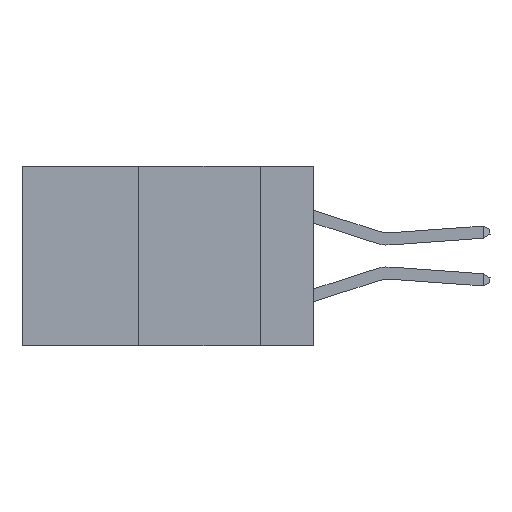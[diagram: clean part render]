
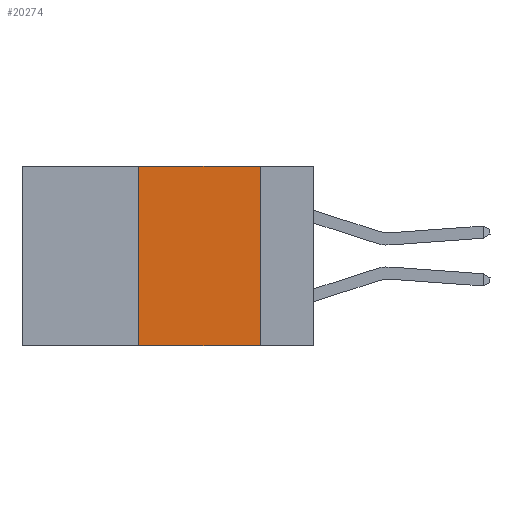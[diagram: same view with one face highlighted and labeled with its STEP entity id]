
A CAD part, left-side view. The second image highlights one B-rep face of the part: STEP entity #20274.
In plain terms, the highlighted planar face has unit normal (-1, 0, 0).
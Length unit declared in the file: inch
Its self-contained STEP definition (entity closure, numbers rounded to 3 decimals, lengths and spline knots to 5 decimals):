
#1145 = FACE_OUTER_BOUND ( 'NONE', #20582, .T. ) ;
#2050 = VERTEX_POINT ( 'NONE', #13366 ) ;
#3745 = ORIENTED_EDGE ( 'NONE', *, *, #16689, .F. ) ;
#4693 = LINE ( 'NONE', #27368, #33928 ) ;
#4699 = EDGE_CURVE ( 'NONE', #14085, #8470, #4693, .T. ) ;
#4722 = VECTOR ( 'NONE', #23053, 39.37008 ) ;
#7476 = CARTESIAN_POINT ( 'NONE',  ( 0., 0.11, 0. ) ) ;
#8258 = PLANE ( 'NONE',  #18762 ) ;
#8470 = VERTEX_POINT ( 'NONE', #16312 ) ;
#10323 = VECTOR ( 'NONE', #19302, 39.37008 ) ;
#13366 = CARTESIAN_POINT ( 'NONE',  ( 0., 0.11, 0. ) ) ;
#14085 = VERTEX_POINT ( 'NONE', #34231 ) ;
#14218 = CARTESIAN_POINT ( 'NONE',  ( 0., 0.6, 0. ) ) ;
#15478 = LINE ( 'NONE', #20334, #10323 ) ;
#15614 = LINE ( 'NONE', #22659, #30700 ) ;
#16303 = EDGE_CURVE ( 'NONE', #36599, #2050, #15614, .T. ) ;
#16312 = CARTESIAN_POINT ( 'NONE',  ( 0., 0.11, -0.37 ) ) ;
#16689 = EDGE_CURVE ( 'NONE', #2050, #8470, #35361, .T. ) ;
#18762 = AXIS2_PLACEMENT_3D ( 'NONE', #14218, #32512, #35388 ) ;
#19302 = DIRECTION ( 'NONE',  ( 0., 0., 1. ) ) ;
#20274 = ADVANCED_FACE ( 'NONE', ( #1145 ), #8258, .F. ) ;
#20334 = CARTESIAN_POINT ( 'NONE',  ( 0., 0.36, 0. ) ) ;
#20582 = EDGE_LOOP ( 'NONE', ( #3745, #25035, #38592, #24503 ) ) ;
#20878 = DIRECTION ( 'NONE',  ( 0., -1., 0. ) ) ;
#22211 = EDGE_CURVE ( 'NONE', #14085, #36599, #15478, .T. ) ;
#22659 = CARTESIAN_POINT ( 'NONE',  ( 0., 0.6, 0. ) ) ;
#22759 = CARTESIAN_POINT ( 'NONE',  ( 0., 0.36, 0. ) ) ;
#23053 = DIRECTION ( 'NONE',  ( 0., 0., -1. ) ) ;
#24503 = ORIENTED_EDGE ( 'NONE', *, *, #4699, .T. ) ;
#25035 = ORIENTED_EDGE ( 'NONE', *, *, #16303, .F. ) ;
#27368 = CARTESIAN_POINT ( 'NONE',  ( 0., 0.6, -0.37 ) ) ;
#28794 = DIRECTION ( 'NONE',  ( 0., -1., 0. ) ) ;
#30700 = VECTOR ( 'NONE', #28794, 39.37008 ) ;
#32512 = DIRECTION ( 'NONE',  ( 1., 0., 0. ) ) ;
#33928 = VECTOR ( 'NONE', #20878, 39.37008 ) ;
#34231 = CARTESIAN_POINT ( 'NONE',  ( 0., 0.36, -0.37 ) ) ;
#35361 = LINE ( 'NONE', #7476, #4722 ) ;
#35388 = DIRECTION ( 'NONE',  ( 0., 0., -1. ) ) ;
#36599 = VERTEX_POINT ( 'NONE', #22759 ) ;
#38592 = ORIENTED_EDGE ( 'NONE', *, *, #22211, .F. ) ;
